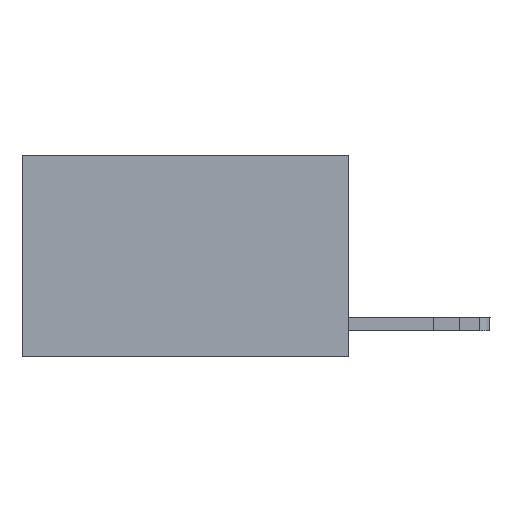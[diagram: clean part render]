
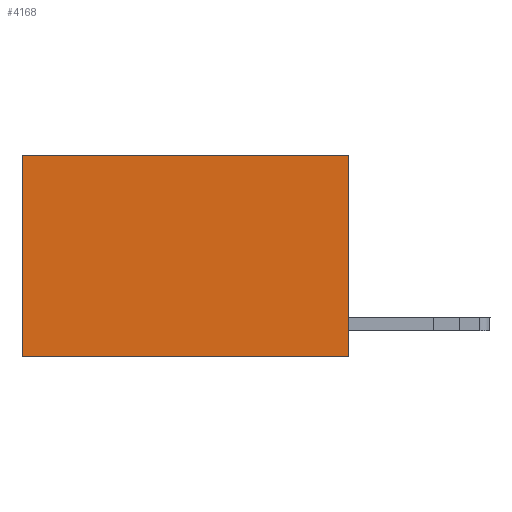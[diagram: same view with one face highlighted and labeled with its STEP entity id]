
A CAD part, left-side view. The second image highlights one B-rep face of the part: STEP entity #4168.
In plain terms, the highlighted planar face has unit normal (-1, 0, 0).
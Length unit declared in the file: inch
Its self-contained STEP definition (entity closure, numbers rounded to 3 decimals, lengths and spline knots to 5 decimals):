
#509 = DIRECTION ( 'NONE',  ( 0., 0., -1. ) ) ;
#611 = CARTESIAN_POINT ( 'NONE',  ( 0.2625, 0.6, 0. ) ) ;
#772 = CARTESIAN_POINT ( 'NONE',  ( 0.2625, 0.6, 0. ) ) ;
#2721 = CARTESIAN_POINT ( 'NONE',  ( 0.2625, 0., 0. ) ) ;
#3877 = VECTOR ( 'NONE', #14675, 39.37008 ) ;
#4126 = VECTOR ( 'NONE', #11664, 39.37008 ) ;
#4168 = ADVANCED_FACE ( 'NONE', ( #9604 ), #13802, .F. ) ;
#4641 = VECTOR ( 'NONE', #6205, 39.37008 ) ;
#4837 = CARTESIAN_POINT ( 'NONE',  ( 0.2625, 0., -0.37 ) ) ;
#5557 = CARTESIAN_POINT ( 'NONE',  ( 0.2625, 0., 0. ) ) ;
#6182 = EDGE_CURVE ( 'NONE', #11363, #12111, #15029, .T. ) ;
#6205 = DIRECTION ( 'NONE',  ( 0., 1., 0. ) ) ;
#6271 = ORIENTED_EDGE ( 'NONE', *, *, #15052, .T. ) ;
#6595 = CARTESIAN_POINT ( 'NONE',  ( 0.2625, 0., -0.37 ) ) ;
#6775 = AXIS2_PLACEMENT_3D ( 'NONE', #15022, #8707, #509 ) ;
#7049 = ORIENTED_EDGE ( 'NONE', *, *, #7889, .F. ) ;
#7728 = LINE ( 'NONE', #16549, #4126 ) ;
#7889 = EDGE_CURVE ( 'NONE', #8061, #11363, #7728, .T. ) ;
#8061 = VERTEX_POINT ( 'NONE', #2721 ) ;
#8237 = EDGE_LOOP ( 'NONE', ( #11072, #12528, #7049, #6271 ) ) ;
#8254 = CARTESIAN_POINT ( 'NONE',  ( 0.2625, 0.6, -0.37 ) ) ;
#8707 = DIRECTION ( 'NONE',  ( 1., 0., 0. ) ) ;
#9604 = FACE_OUTER_BOUND ( 'NONE', #8237, .T. ) ;
#10277 = DIRECTION ( 'NONE',  ( 0., 0., -1. ) ) ;
#10996 = VECTOR ( 'NONE', #10277, 39.37008 ) ;
#11028 = LINE ( 'NONE', #5557, #3877 ) ;
#11072 = ORIENTED_EDGE ( 'NONE', *, *, #16244, .T. ) ;
#11363 = VERTEX_POINT ( 'NONE', #6595 ) ;
#11664 = DIRECTION ( 'NONE',  ( 0., 0., -1. ) ) ;
#12111 = VERTEX_POINT ( 'NONE', #8254 ) ;
#12528 = ORIENTED_EDGE ( 'NONE', *, *, #6182, .F. ) ;
#13802 = PLANE ( 'NONE',  #6775 ) ;
#14675 = DIRECTION ( 'NONE',  ( 0., 1., 0. ) ) ;
#15022 = CARTESIAN_POINT ( 'NONE',  ( 0.2625, 0., 0. ) ) ;
#15029 = LINE ( 'NONE', #4837, #4641 ) ;
#15052 = EDGE_CURVE ( 'NONE', #8061, #15347, #11028, .T. ) ;
#15347 = VERTEX_POINT ( 'NONE', #611 ) ;
#16244 = EDGE_CURVE ( 'NONE', #15347, #12111, #16777, .T. ) ;
#16549 = CARTESIAN_POINT ( 'NONE',  ( 0.2625, 0., 0. ) ) ;
#16777 = LINE ( 'NONE', #772, #10996 ) ;
